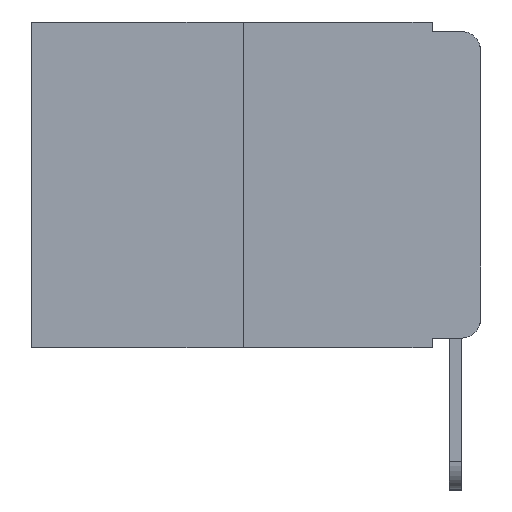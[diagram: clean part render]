
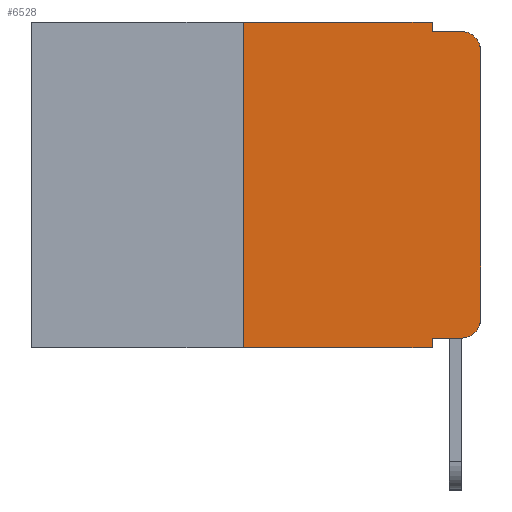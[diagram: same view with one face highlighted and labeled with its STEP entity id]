
A CAD part, left-side view. The second image highlights one B-rep face of the part: STEP entity #6528.
In plain terms, the highlighted planar face has unit normal (-1, 0, 0).
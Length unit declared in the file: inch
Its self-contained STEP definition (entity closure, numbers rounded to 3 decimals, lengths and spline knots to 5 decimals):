
#45 = VECTOR ( 'NONE', #5122, 39.37008 ) ;
#299 = DIRECTION ( 'NONE',  ( 0., 0., -1. ) ) ;
#488 = LINE ( 'NONE', #868, #1461 ) ;
#491 = LINE ( 'NONE', #2589, #9474 ) ;
#544 = DIRECTION ( 'NONE',  ( 0., 0., -1. ) ) ;
#706 = EDGE_LOOP ( 'NONE', ( #8107, #13131, #14642, #12746, #13007, #15221, #13364, #15587, #1845, #3415 ) ) ;
#814 = DIRECTION ( 'NONE',  ( 0., -1., 0. ) ) ;
#868 = CARTESIAN_POINT ( 'NONE',  ( 0., 0.051, 0. ) ) ;
#1006 = CARTESIAN_POINT ( 'NONE',  ( 0., 0., -0.313 ) ) ;
#1185 = AXIS2_PLACEMENT_3D ( 'NONE', #9199, #10481, #544 ) ;
#1294 = CARTESIAN_POINT ( 'NONE',  ( 0., 0.25, 0. ) ) ;
#1461 = VECTOR ( 'NONE', #14593, 39.37008 ) ;
#1480 = VERTEX_POINT ( 'NONE', #3942 ) ;
#1845 = ORIENTED_EDGE ( 'NONE', *, *, #2297, .T. ) ;
#1896 = CARTESIAN_POINT ( 'NONE',  ( 0., 0.051, -0.333 ) ) ;
#2094 = CARTESIAN_POINT ( 'NONE',  ( 0., 0.25, 0. ) ) ;
#2297 = EDGE_CURVE ( 'NONE', #12375, #12654, #2509, .T. ) ;
#2309 = VERTEX_POINT ( 'NONE', #2094 ) ;
#2509 = LINE ( 'NONE', #1896, #9726 ) ;
#2589 = CARTESIAN_POINT ( 'NONE',  ( 0., 0.051, 0. ) ) ;
#2706 = VERTEX_POINT ( 'NONE', #1006 ) ;
#3415 = ORIENTED_EDGE ( 'NONE', *, *, #9470, .T. ) ;
#3587 = DIRECTION ( 'NONE',  ( 0., 0., 1. ) ) ;
#3668 = CARTESIAN_POINT ( 'NONE',  ( 0., 0.02, -0.01 ) ) ;
#3942 = CARTESIAN_POINT ( 'NONE',  ( 0., 0., -0.03 ) ) ;
#4547 = CARTESIAN_POINT ( 'NONE',  ( 0., 0.473, 0. ) ) ;
#4713 = EDGE_CURVE ( 'NONE', #11867, #12170, #491, .T. ) ;
#4855 = CARTESIAN_POINT ( 'NONE',  ( 0., 0.051, -0.01 ) ) ;
#5012 = CARTESIAN_POINT ( 'NONE',  ( 0., 0.473, -0.343 ) ) ;
#5122 = DIRECTION ( 'NONE',  ( 0., -1., 0. ) ) ;
#5173 = LINE ( 'NONE', #6144, #15130 ) ;
#5282 = EDGE_CURVE ( 'NONE', #1480, #12200, #6274, .T. ) ;
#5386 = CARTESIAN_POINT ( 'NONE',  ( 0., 0.051, 0. ) ) ;
#5491 = VERTEX_POINT ( 'NONE', #9382 ) ;
#6054 = VECTOR ( 'NONE', #10484, 39.37008 ) ;
#6144 = CARTESIAN_POINT ( 'NONE',  ( 0., 0., 0. ) ) ;
#6146 = DIRECTION ( 'NONE',  ( 0., 0., -1. ) ) ;
#6186 = AXIS2_PLACEMENT_3D ( 'NONE', #6558, #12711, #299 ) ;
#6274 = CIRCLE ( 'NONE', #1185, 0.02 ) ;
#6276 = CARTESIAN_POINT ( 'NONE',  ( 0., 0.051, -0.333 ) ) ;
#6528 = ADVANCED_FACE ( 'NONE', ( #8205 ), #11248, .F. ) ;
#6558 = CARTESIAN_POINT ( 'NONE',  ( 0., 0.02, -0.313 ) ) ;
#6614 = LINE ( 'NONE', #5012, #45 ) ;
#6956 = DIRECTION ( 'NONE',  ( 0., -1., 0. ) ) ;
#7302 = LINE ( 'NONE', #1294, #10669 ) ;
#7407 = DIRECTION ( 'NONE',  ( 0., 0., 1. ) ) ;
#8107 = ORIENTED_EDGE ( 'NONE', *, *, #8775, .T. ) ;
#8205 = FACE_OUTER_BOUND ( 'NONE', #706, .T. ) ;
#8775 = EDGE_CURVE ( 'NONE', #2706, #1480, #5173, .T. ) ;
#8804 = EDGE_CURVE ( 'NONE', #5491, #2309, #7302, .T. ) ;
#9199 = CARTESIAN_POINT ( 'NONE',  ( 0., 0.02, -0.03 ) ) ;
#9263 = EDGE_CURVE ( 'NONE', #12375, #10555, #488, .T. ) ;
#9382 = CARTESIAN_POINT ( 'NONE',  ( 0., 0.25, -0.343 ) ) ;
#9470 = EDGE_CURVE ( 'NONE', #12654, #2706, #12963, .T. ) ;
#9474 = VECTOR ( 'NONE', #6146, 39.37008 ) ;
#9593 = LINE ( 'NONE', #4547, #12902 ) ;
#9726 = VECTOR ( 'NONE', #814, 39.37008 ) ;
#10240 = EDGE_CURVE ( 'NONE', #12170, #12200, #15460, .T. ) ;
#10481 = DIRECTION ( 'NONE',  ( -1., 0., 0. ) ) ;
#10484 = DIRECTION ( 'NONE',  ( 0., -1., 0. ) ) ;
#10555 = VERTEX_POINT ( 'NONE', #12045 ) ;
#10669 = VECTOR ( 'NONE', #7407, 39.37008 ) ;
#10869 = EDGE_CURVE ( 'NONE', #2309, #11867, #9593, .T. ) ;
#11145 = CARTESIAN_POINT ( 'NONE',  ( 0., 0.473, 0. ) ) ;
#11164 = EDGE_CURVE ( 'NONE', #5491, #10555, #6614, .T. ) ;
#11248 = PLANE ( 'NONE',  #13808 ) ;
#11867 = VERTEX_POINT ( 'NONE', #5386 ) ;
#12045 = CARTESIAN_POINT ( 'NONE',  ( 0., 0.051, -0.343 ) ) ;
#12170 = VERTEX_POINT ( 'NONE', #4855 ) ;
#12200 = VERTEX_POINT ( 'NONE', #3668 ) ;
#12375 = VERTEX_POINT ( 'NONE', #6276 ) ;
#12527 = DIRECTION ( 'NONE',  ( 1., 0., 0. ) ) ;
#12654 = VERTEX_POINT ( 'NONE', #13238 ) ;
#12711 = DIRECTION ( 'NONE',  ( -1., 0., 0. ) ) ;
#12746 = ORIENTED_EDGE ( 'NONE', *, *, #4713, .F. ) ;
#12902 = VECTOR ( 'NONE', #6956, 39.37008 ) ;
#12963 = CIRCLE ( 'NONE', #6186, 0.02 ) ;
#13007 = ORIENTED_EDGE ( 'NONE', *, *, #10869, .F. ) ;
#13131 = ORIENTED_EDGE ( 'NONE', *, *, #5282, .T. ) ;
#13238 = CARTESIAN_POINT ( 'NONE',  ( 0., 0.02, -0.333 ) ) ;
#13364 = ORIENTED_EDGE ( 'NONE', *, *, #11164, .T. ) ;
#13614 = DIRECTION ( 'NONE',  ( 0., 0., -1. ) ) ;
#13808 = AXIS2_PLACEMENT_3D ( 'NONE', #11145, #12527, #13614 ) ;
#14593 = DIRECTION ( 'NONE',  ( 0., 0., -1. ) ) ;
#14642 = ORIENTED_EDGE ( 'NONE', *, *, #10240, .F. ) ;
#15130 = VECTOR ( 'NONE', #3587, 39.37008 ) ;
#15221 = ORIENTED_EDGE ( 'NONE', *, *, #8804, .F. ) ;
#15460 = LINE ( 'NONE', #15649, #6054 ) ;
#15587 = ORIENTED_EDGE ( 'NONE', *, *, #9263, .F. ) ;
#15649 = CARTESIAN_POINT ( 'NONE',  ( 0., 0.051, -0.01 ) ) ;
